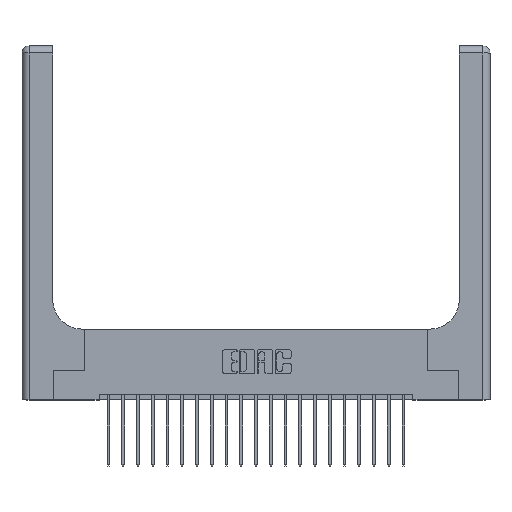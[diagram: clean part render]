
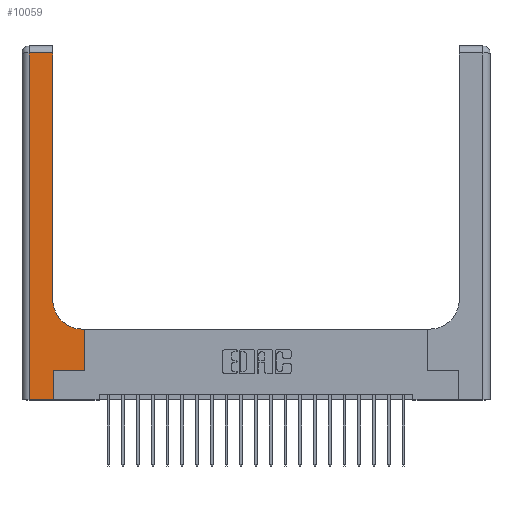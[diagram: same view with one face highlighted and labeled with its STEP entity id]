
A CAD part, top view. The second image highlights one B-rep face of the part: STEP entity #10059.
In plain terms, the highlighted planar face has unit normal (0, 0, 1).
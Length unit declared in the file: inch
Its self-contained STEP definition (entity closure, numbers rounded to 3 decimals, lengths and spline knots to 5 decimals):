
#315 = VECTOR ( 'NONE', #3854, 39.37008 ) ;
#672 = VECTOR ( 'NONE', #1440, 39.37008 ) ;
#872 = EDGE_CURVE ( 'NONE', #13285, #6137, #12251, .T. ) ;
#1051 = LINE ( 'NONE', #12550, #20223 ) ;
#1258 = FACE_OUTER_BOUND ( 'NONE', #9366, .T. ) ;
#1440 = DIRECTION ( 'NONE',  ( -1., 0., 0. ) ) ;
#2069 = LINE ( 'NONE', #21347, #15211 ) ;
#2269 = VECTOR ( 'NONE', #11671, 39.37008 ) ;
#2745 = CARTESIAN_POINT ( 'NONE',  ( 0.528, 0.25, 0.37 ) ) ;
#3117 = VECTOR ( 'NONE', #13142, 39.37008 ) ;
#3214 = VECTOR ( 'NONE', #15107, 39.37008 ) ;
#3227 = CARTESIAN_POINT ( 'NONE',  ( 0., 3., 0.37 ) ) ;
#3347 = VERTEX_POINT ( 'NONE', #6830 ) ;
#3843 = EDGE_CURVE ( 'NONE', #17089, #10990, #6371, .T. ) ;
#3854 = DIRECTION ( 'NONE',  ( 0., 1., 0. ) ) ;
#3888 = DIRECTION ( 'NONE',  ( 0., -1., 0. ) ) ;
#3931 = CARTESIAN_POINT ( 'NONE',  ( 0.528, 0.25, 0.37 ) ) ;
#5315 = AXIS2_PLACEMENT_3D ( 'NONE', #9815, #6378, #14817 ) ;
#6137 = VERTEX_POINT ( 'NONE', #10999 ) ;
#6371 = CIRCLE ( 'NONE', #5315, 0.25 ) ;
#6378 = DIRECTION ( 'NONE',  ( 0., 0., -1. ) ) ;
#6413 = EDGE_CURVE ( 'NONE', #10990, #3347, #14702, .T. ) ;
#6607 = CARTESIAN_POINT ( 'NONE',  ( 0., 0., 0.37 ) ) ;
#6830 = CARTESIAN_POINT ( 'NONE',  ( 0.26, 2.94, 0.37 ) ) ;
#6980 = EDGE_CURVE ( 'NONE', #6137, #17223, #21355, .T. ) ;
#8211 = CARTESIAN_POINT ( 'NONE',  ( 0.528, 0.6, 0.37 ) ) ;
#8699 = VECTOR ( 'NONE', #16271, 39.37008 ) ;
#9366 = EDGE_LOOP ( 'NONE', ( #20698, #12109, #16602, #18306, #17476, #15497, #17173, #14507, #19413 ) ) ;
#9475 = CARTESIAN_POINT ( 'NONE',  ( 0.51, 0.6, 0.37 ) ) ;
#9681 = VERTEX_POINT ( 'NONE', #20566 ) ;
#9815 = CARTESIAN_POINT ( 'NONE',  ( 0.51, 0.85, 0.37 ) ) ;
#10059 = ADVANCED_FACE ( 'NONE', ( #1258 ), #13293, .F. ) ;
#10102 = CARTESIAN_POINT ( 'NONE',  ( 0.26, 3., 0.37 ) ) ;
#10123 = CARTESIAN_POINT ( 'NONE',  ( 0.265, 0., 0.37 ) ) ;
#10990 = VERTEX_POINT ( 'NONE', #21093 ) ;
#10999 = CARTESIAN_POINT ( 'NONE',  ( 0.265, 0.25, 0.37 ) ) ;
#11194 = DIRECTION ( 'NONE',  ( -1., 0., 0. ) ) ;
#11502 = CARTESIAN_POINT ( 'NONE',  ( 0., 2.94, 0.37 ) ) ;
#11671 = DIRECTION ( 'NONE',  ( 0., 1., 0. ) ) ;
#12109 = ORIENTED_EDGE ( 'NONE', *, *, #20491, .T. ) ;
#12251 = LINE ( 'NONE', #10123, #2269 ) ;
#12550 = CARTESIAN_POINT ( 'NONE',  ( 0.06, 3., 0.37 ) ) ;
#13142 = DIRECTION ( 'NONE',  ( 0., 1., 0. ) ) ;
#13285 = VERTEX_POINT ( 'NONE', #19545 ) ;
#13293 = PLANE ( 'NONE',  #17222 ) ;
#13874 = EDGE_CURVE ( 'NONE', #18783, #13285, #17410, .T. ) ;
#13891 = VERTEX_POINT ( 'NONE', #8211 ) ;
#14507 = ORIENTED_EDGE ( 'NONE', *, *, #17286, .T. ) ;
#14702 = LINE ( 'NONE', #10102, #3117 ) ;
#14817 = DIRECTION ( 'NONE',  ( 1., 0., 0. ) ) ;
#14992 = DIRECTION ( 'NONE',  ( 0., 0., -1. ) ) ;
#15107 = DIRECTION ( 'NONE',  ( 1., 0., 0. ) ) ;
#15211 = VECTOR ( 'NONE', #11194, 39.37008 ) ;
#15497 = ORIENTED_EDGE ( 'NONE', *, *, #6980, .T. ) ;
#15663 = EDGE_CURVE ( 'NONE', #17223, #13891, #17664, .T. ) ;
#16271 = DIRECTION ( 'NONE',  ( 1., 0., 0. ) ) ;
#16555 = CARTESIAN_POINT ( 'NONE',  ( 0.265, 0.25, 0.37 ) ) ;
#16602 = ORIENTED_EDGE ( 'NONE', *, *, #16953, .T. ) ;
#16666 = DIRECTION ( 'NONE',  ( -1., 0., 0. ) ) ;
#16917 = CARTESIAN_POINT ( 'NONE',  ( 0.06, 0., 0.37 ) ) ;
#16953 = EDGE_CURVE ( 'NONE', #9681, #18783, #1051, .T. ) ;
#17089 = VERTEX_POINT ( 'NONE', #9475 ) ;
#17173 = ORIENTED_EDGE ( 'NONE', *, *, #15663, .T. ) ;
#17222 = AXIS2_PLACEMENT_3D ( 'NONE', #3227, #14992, #16666 ) ;
#17223 = VERTEX_POINT ( 'NONE', #2745 ) ;
#17286 = EDGE_CURVE ( 'NONE', #13891, #17089, #2069, .T. ) ;
#17410 = LINE ( 'NONE', #6607, #3214 ) ;
#17476 = ORIENTED_EDGE ( 'NONE', *, *, #872, .T. ) ;
#17664 = LINE ( 'NONE', #3931, #315 ) ;
#18306 = ORIENTED_EDGE ( 'NONE', *, *, #13874, .T. ) ;
#18542 = LINE ( 'NONE', #11502, #672 ) ;
#18783 = VERTEX_POINT ( 'NONE', #16917 ) ;
#19413 = ORIENTED_EDGE ( 'NONE', *, *, #3843, .T. ) ;
#19545 = CARTESIAN_POINT ( 'NONE',  ( 0.265, 0., 0.37 ) ) ;
#20223 = VECTOR ( 'NONE', #3888, 39.37008 ) ;
#20491 = EDGE_CURVE ( 'NONE', #3347, #9681, #18542, .T. ) ;
#20566 = CARTESIAN_POINT ( 'NONE',  ( 0.06, 2.94, 0.37 ) ) ;
#20698 = ORIENTED_EDGE ( 'NONE', *, *, #6413, .T. ) ;
#21093 = CARTESIAN_POINT ( 'NONE',  ( 0.26, 0.85, 0.37 ) ) ;
#21347 = CARTESIAN_POINT ( 'NONE',  ( 0.26, 0.6, 0.37 ) ) ;
#21355 = LINE ( 'NONE', #16555, #8699 ) ;
